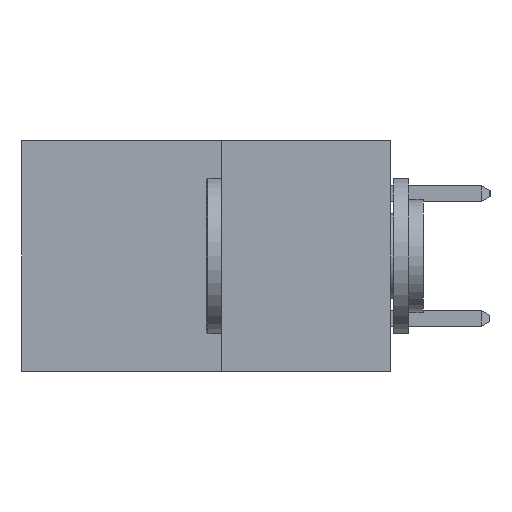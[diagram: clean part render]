
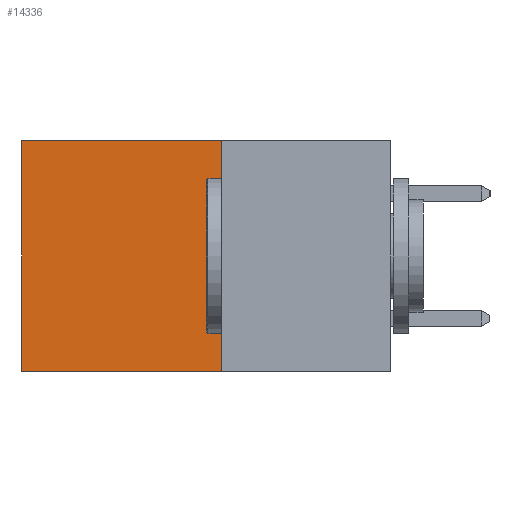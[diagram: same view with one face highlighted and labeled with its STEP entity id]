
A CAD part, left-side view. The second image highlights one B-rep face of the part: STEP entity #14336.
In plain terms, the highlighted planar face has unit normal (-1, 0, 0).
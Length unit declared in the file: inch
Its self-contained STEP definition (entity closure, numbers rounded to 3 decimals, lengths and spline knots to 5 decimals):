
#1071 = LINE ( 'NONE', #7408, #13568 ) ;
#1709 = EDGE_CURVE ( 'NONE', #12613, #10195, #8085, .T. ) ;
#2044 = ORIENTED_EDGE ( 'NONE', *, *, #8080, .T. ) ;
#2684 = VERTEX_POINT ( 'NONE', #5991 ) ;
#3219 = VECTOR ( 'NONE', #7989, 39.37008 ) ;
#3372 = DIRECTION ( 'NONE',  ( 0., 0., -1. ) ) ;
#3547 = EDGE_CURVE ( 'NONE', #12613, #2684, #8781, .T. ) ;
#5991 = CARTESIAN_POINT ( 'NONE',  ( 0.277, 0.27, -0.37 ) ) ;
#6298 = DIRECTION ( 'NONE',  ( 0., 1., 0. ) ) ;
#6317 = LINE ( 'NONE', #11414, #3219 ) ;
#6587 = ORIENTED_EDGE ( 'NONE', *, *, #1709, .T. ) ;
#6822 = PLANE ( 'NONE',  #13208 ) ;
#7408 = CARTESIAN_POINT ( 'NONE',  ( 0.277, 0.27, -0.37 ) ) ;
#7989 = DIRECTION ( 'NONE',  ( 0., 0., -1. ) ) ;
#8080 = EDGE_CURVE ( 'NONE', #10195, #9106, #6317, .T. ) ;
#8085 = LINE ( 'NONE', #9663, #8453 ) ;
#8453 = VECTOR ( 'NONE', #11880, 39.37008 ) ;
#8781 = LINE ( 'NONE', #10803, #14420 ) ;
#9106 = VERTEX_POINT ( 'NONE', #14342 ) ;
#9663 = CARTESIAN_POINT ( 'NONE',  ( 0.277, 0.27, 0. ) ) ;
#9715 = EDGE_CURVE ( 'NONE', #2684, #9106, #1071, .T. ) ;
#10195 = VERTEX_POINT ( 'NONE', #13888 ) ;
#10198 = DIRECTION ( 'NONE',  ( 0., 0., -1. ) ) ;
#10308 = DIRECTION ( 'NONE',  ( 1., 0., 0. ) ) ;
#10803 = CARTESIAN_POINT ( 'NONE',  ( 0.277, 0.27, -0.37 ) ) ;
#11031 = CARTESIAN_POINT ( 'NONE',  ( 0.277, 0.27, 0. ) ) ;
#11414 = CARTESIAN_POINT ( 'NONE',  ( 0.277, 0.59, -0.37 ) ) ;
#11880 = DIRECTION ( 'NONE',  ( 0., 1., 0. ) ) ;
#12613 = VERTEX_POINT ( 'NONE', #11031 ) ;
#12621 = EDGE_LOOP ( 'NONE', ( #2044, #13357, #12839, #6587 ) ) ;
#12839 = ORIENTED_EDGE ( 'NONE', *, *, #3547, .F. ) ;
#13208 = AXIS2_PLACEMENT_3D ( 'NONE', #14678, #10308, #3372 ) ;
#13357 = ORIENTED_EDGE ( 'NONE', *, *, #9715, .F. ) ;
#13468 = FACE_OUTER_BOUND ( 'NONE', #12621, .T. ) ;
#13568 = VECTOR ( 'NONE', #6298, 39.37008 ) ;
#13888 = CARTESIAN_POINT ( 'NONE',  ( 0.277, 0.59, 0. ) ) ;
#14336 = ADVANCED_FACE ( 'NONE', ( #13468 ), #6822, .F. ) ;
#14342 = CARTESIAN_POINT ( 'NONE',  ( 0.277, 0.59, -0.37 ) ) ;
#14420 = VECTOR ( 'NONE', #10198, 39.37008 ) ;
#14678 = CARTESIAN_POINT ( 'NONE',  ( 0.277, 0.27, -0.37 ) ) ;
